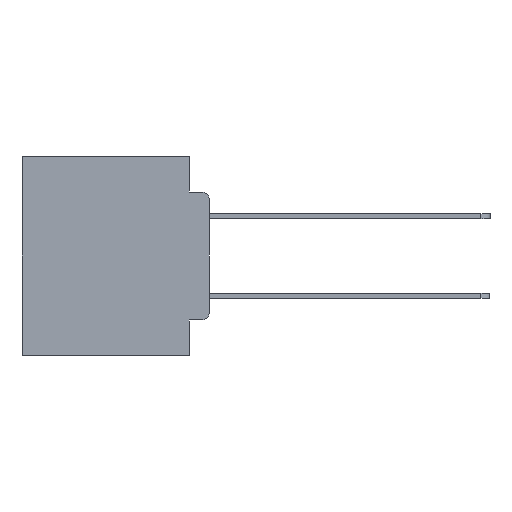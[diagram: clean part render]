
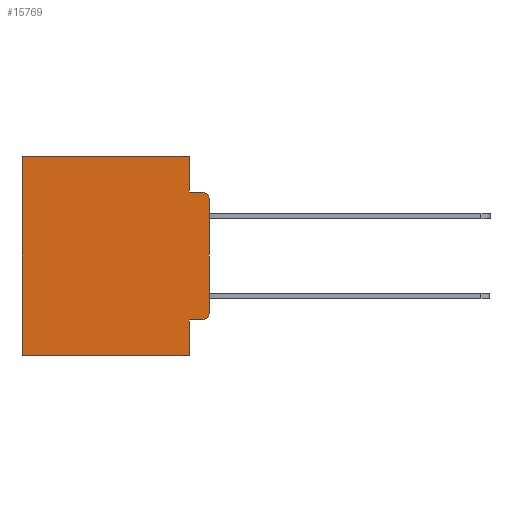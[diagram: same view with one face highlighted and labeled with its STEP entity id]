
A CAD part, left-side view. The second image highlights one B-rep face of the part: STEP entity #15769.
In plain terms, the highlighted planar face has unit normal (-1, 0, 0).
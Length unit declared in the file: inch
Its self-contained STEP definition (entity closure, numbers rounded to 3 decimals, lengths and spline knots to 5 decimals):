
#804 = VERTEX_POINT ( 'NONE', #18167 ) ;
#1196 = EDGE_CURVE ( 'NONE', #14335, #8031, #17468, .T. ) ;
#1312 = EDGE_CURVE ( 'NONE', #16625, #21374, #9413, .T. ) ;
#1826 = CARTESIAN_POINT ( 'NONE',  ( 0.298, 0., 0. ) ) ;
#1904 = LINE ( 'NONE', #5144, #25071 ) ;
#2159 = CARTESIAN_POINT ( 'NONE',  ( 0.298, 0., -0.5 ) ) ;
#2513 = DIRECTION ( 'NONE',  ( 0., -1., 0. ) ) ;
#2877 = AXIS2_PLACEMENT_3D ( 'NONE', #1826, #4115, #19847 ) ;
#2958 = ORIENTED_EDGE ( 'NONE', *, *, #1196, .T. ) ;
#3039 = CARTESIAN_POINT ( 'NONE',  ( 0.298, 0.473, -0.5 ) ) ;
#4115 = DIRECTION ( 'NONE',  ( 1., 0., 0. ) ) ;
#4447 = DIRECTION ( 'NONE',  ( 0., 1., 0. ) ) ;
#4812 = CARTESIAN_POINT ( 'NONE',  ( 0.298, 0.051, -0.0885 ) ) ;
#4858 = ORIENTED_EDGE ( 'NONE', *, *, #5294, .T. ) ;
#5144 = CARTESIAN_POINT ( 'NONE',  ( 0.298, 0.051, -0.4115 ) ) ;
#5294 = EDGE_CURVE ( 'NONE', #20673, #28570, #1904, .T. ) ;
#5698 = AXIS2_PLACEMENT_3D ( 'NONE', #26984, #9983, #26003 ) ;
#5912 = LINE ( 'NONE', #4812, #28872 ) ;
#6411 = DIRECTION ( 'NONE',  ( 0., 1., 0. ) ) ;
#7144 = CARTESIAN_POINT ( 'NONE',  ( 0.298, 0.051, -0.4115 ) ) ;
#7223 = CARTESIAN_POINT ( 'NONE',  ( 0.298, 0.02, -0.4115 ) ) ;
#7680 = VECTOR ( 'NONE', #28045, 39.37008 ) ;
#8031 = VERTEX_POINT ( 'NONE', #3039 ) ;
#8131 = LINE ( 'NONE', #18203, #25219 ) ;
#8415 = VECTOR ( 'NONE', #6411, 39.37008 ) ;
#8772 = DIRECTION ( 'NONE',  ( 0., 0., -1. ) ) ;
#9049 = CARTESIAN_POINT ( 'NONE',  ( 0.298, 0., 0. ) ) ;
#9413 = CIRCLE ( 'NONE', #5698, 0.02 ) ;
#9621 = EDGE_LOOP ( 'NONE', ( #14639, #13882, #23125, #11973, #17185, #2958, #28444, #24698, #4858, #11459 ) ) ;
#9983 = DIRECTION ( 'NONE',  ( -1., 0., 0. ) ) ;
#10447 = EDGE_CURVE ( 'NONE', #804, #21374, #5912, .T. ) ;
#10906 = CARTESIAN_POINT ( 'NONE',  ( 0.298, 0.02, -0.3915 ) ) ;
#11369 = CARTESIAN_POINT ( 'NONE',  ( 0.298, 0., -0.1085 ) ) ;
#11459 = ORIENTED_EDGE ( 'NONE', *, *, #17784, .T. ) ;
#11973 = ORIENTED_EDGE ( 'NONE', *, *, #17054, .F. ) ;
#12115 = VECTOR ( 'NONE', #8772, 39.37008 ) ;
#13553 = DIRECTION ( 'NONE',  ( 0., 0., -1. ) ) ;
#13589 = VECTOR ( 'NONE', #24851, 39.37008 ) ;
#13882 = ORIENTED_EDGE ( 'NONE', *, *, #1312, .T. ) ;
#14205 = DIRECTION ( 'NONE',  ( 0., -1., 0. ) ) ;
#14335 = VERTEX_POINT ( 'NONE', #23790 ) ;
#14639 = ORIENTED_EDGE ( 'NONE', *, *, #19998, .F. ) ;
#14936 = CARTESIAN_POINT ( 'NONE',  ( 0.298, 0.051, 0. ) ) ;
#15357 = PLANE ( 'NONE',  #2877 ) ;
#15769 = ADVANCED_FACE ( 'NONE', ( #22490 ), #15357, .F. ) ;
#16625 = VERTEX_POINT ( 'NONE', #11369 ) ;
#17054 = EDGE_CURVE ( 'NONE', #22764, #804, #23947, .T. ) ;
#17177 = CIRCLE ( 'NONE', #25102, 0.02 ) ;
#17185 = ORIENTED_EDGE ( 'NONE', *, *, #25706, .T. ) ;
#17468 = LINE ( 'NONE', #26188, #7680 ) ;
#17584 = CARTESIAN_POINT ( 'NONE',  ( 0.298, 0., 0. ) ) ;
#17784 = EDGE_CURVE ( 'NONE', #28570, #22940, #17177, .T. ) ;
#18167 = CARTESIAN_POINT ( 'NONE',  ( 0.298, 0.051, -0.0885 ) ) ;
#18203 = CARTESIAN_POINT ( 'NONE',  ( 0.298, 0.051, 0. ) ) ;
#18405 = EDGE_CURVE ( 'NONE', #28270, #8031, #21373, .T. ) ;
#19528 = LINE ( 'NONE', #9049, #13589 ) ;
#19847 = DIRECTION ( 'NONE',  ( 0., 0., -1. ) ) ;
#19998 = EDGE_CURVE ( 'NONE', #16625, #22940, #19528, .T. ) ;
#20541 = DIRECTION ( 'NONE',  ( 0., 0., -1. ) ) ;
#20673 = VERTEX_POINT ( 'NONE', #7144 ) ;
#20785 = CARTESIAN_POINT ( 'NONE',  ( 0.298, 0.02, -0.0885 ) ) ;
#21373 = LINE ( 'NONE', #2159, #27228 ) ;
#21374 = VERTEX_POINT ( 'NONE', #20785 ) ;
#21797 = CARTESIAN_POINT ( 'NONE',  ( 0.298, 0.051, -0.5 ) ) ;
#22490 = FACE_OUTER_BOUND ( 'NONE', #9621, .T. ) ;
#22764 = VERTEX_POINT ( 'NONE', #14936 ) ;
#22940 = VERTEX_POINT ( 'NONE', #24369 ) ;
#23125 = ORIENTED_EDGE ( 'NONE', *, *, #10447, .F. ) ;
#23753 = EDGE_CURVE ( 'NONE', #20673, #28270, #8131, .T. ) ;
#23790 = CARTESIAN_POINT ( 'NONE',  ( 0.298, 0.473, 0. ) ) ;
#23947 = LINE ( 'NONE', #28745, #12115 ) ;
#24369 = CARTESIAN_POINT ( 'NONE',  ( 0.298, 0., -0.3915 ) ) ;
#24698 = ORIENTED_EDGE ( 'NONE', *, *, #23753, .F. ) ;
#24851 = DIRECTION ( 'NONE',  ( 0., 0., -1. ) ) ;
#25071 = VECTOR ( 'NONE', #14205, 39.37008 ) ;
#25102 = AXIS2_PLACEMENT_3D ( 'NONE', #10906, #26472, #13553 ) ;
#25219 = VECTOR ( 'NONE', #20541, 39.37008 ) ;
#25706 = EDGE_CURVE ( 'NONE', #22764, #14335, #26168, .T. ) ;
#26003 = DIRECTION ( 'NONE',  ( 0., 0., -1. ) ) ;
#26168 = LINE ( 'NONE', #17584, #8415 ) ;
#26188 = CARTESIAN_POINT ( 'NONE',  ( 0.298, 0.473, 0. ) ) ;
#26472 = DIRECTION ( 'NONE',  ( -1., 0., 0. ) ) ;
#26984 = CARTESIAN_POINT ( 'NONE',  ( 0.298, 0.02, -0.1085 ) ) ;
#27228 = VECTOR ( 'NONE', #4447, 39.37008 ) ;
#28045 = DIRECTION ( 'NONE',  ( 0., 0., -1. ) ) ;
#28270 = VERTEX_POINT ( 'NONE', #21797 ) ;
#28444 = ORIENTED_EDGE ( 'NONE', *, *, #18405, .F. ) ;
#28570 = VERTEX_POINT ( 'NONE', #7223 ) ;
#28745 = CARTESIAN_POINT ( 'NONE',  ( 0.298, 0.051, 0. ) ) ;
#28872 = VECTOR ( 'NONE', #2513, 39.37008 ) ;
